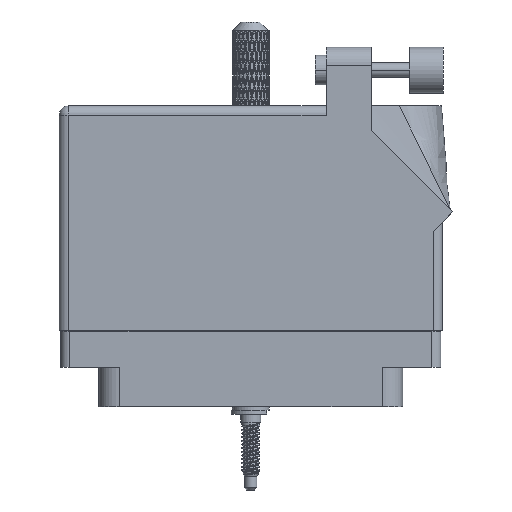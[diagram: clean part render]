
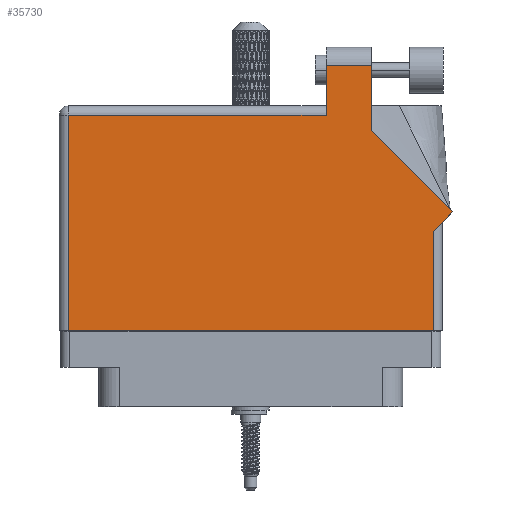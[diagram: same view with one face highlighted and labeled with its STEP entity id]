
A CAD part, front view. The second image highlights one B-rep face of the part: STEP entity #35730.
In plain terms, the highlighted face is planar.
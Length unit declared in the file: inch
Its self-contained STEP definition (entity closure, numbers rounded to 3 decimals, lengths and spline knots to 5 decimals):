
#461 = ORIENTED_EDGE ( 'NONE', *, *, #35735, .T. ) ;
#1427 = LINE ( 'NONE', #69661, #65424 ) ;
#1857 = CARTESIAN_POINT ( 'NONE',  ( -1.244, -0.1, 0.455 ) ) ;
#3035 = CARTESIAN_POINT ( 'NONE',  ( -1.306, 1.43, 0.455 ) ) ;
#3045 = VERTEX_POINT ( 'NONE', #46805 ) ;
#9714 = CARTESIAN_POINT ( 'NONE',  ( 0.513, 1.43, 0.455 ) ) ;
#10929 = VECTOR ( 'NONE', #101242, 39.37008 ) ;
#12456 = CARTESIAN_POINT ( 'NONE',  ( 1.244, 0.637, 0.455 ) ) ;
#15133 = VERTEX_POINT ( 'NONE', #17877 ) ;
#17607 = CARTESIAN_POINT ( 'NONE',  ( 1.37671, 0.70771, 0.455 ) ) ;
#17877 = CARTESIAN_POINT ( 'NONE',  ( 1.244, -0.1, 0.455 ) ) ;
#18217 = ORIENTED_EDGE ( 'NONE', *, *, #37475, .T. ) ;
#20458 = ORIENTED_EDGE ( 'NONE', *, *, #99227, .T. ) ;
#21428 = LINE ( 'NONE', #12456, #99549 ) ;
#21440 = DIRECTION ( 'NONE',  ( 0., 1., 0. ) ) ;
#21801 = LINE ( 'NONE', #76843, #89951 ) ;
#21829 = CARTESIAN_POINT ( 'NONE',  ( 0.82, 1.26442, 0.455 ) ) ;
#22367 = CARTESIAN_POINT ( 'NONE',  ( -1.244, 1.368, 0.455 ) ) ;
#26909 = LINE ( 'NONE', #9714, #49633 ) ;
#35700 = VECTOR ( 'NONE', #84790, 39.37008 ) ;
#35730 = ADVANCED_FACE ( 'NONE', ( #83918 ), #110206, .F. ) ;
#35735 = EDGE_CURVE ( 'NONE', #67840, #49804, #72578, .T. ) ;
#36188 = EDGE_CURVE ( 'NONE', #3045, #116343, #1427, .T. ) ;
#36467 = EDGE_CURVE ( 'NONE', #81797, #103691, #62552, .T. ) ;
#37475 = EDGE_CURVE ( 'NONE', #96140, #67840, #86640, .T. ) ;
#37841 = ORIENTED_EDGE ( 'NONE', *, *, #52600, .T. ) ;
#38624 = EDGE_CURVE ( 'NONE', #116343, #96140, #26909, .T. ) ;
#44451 = ORIENTED_EDGE ( 'NONE', *, *, #36467, .T. ) ;
#46805 = CARTESIAN_POINT ( 'NONE',  ( 0.82, 1.705, 0.455 ) ) ;
#49584 = EDGE_LOOP ( 'NONE', ( #85279, #93292, #104992, #18217, #461, #37841, #75989, #44451, #20458 ) ) ;
#49633 = VECTOR ( 'NONE', #86597, 39.37008 ) ;
#49804 = VERTEX_POINT ( 'NONE', #97692 ) ;
#51833 = LINE ( 'NONE', #21829, #105667 ) ;
#52600 = EDGE_CURVE ( 'NONE', #49804, #15133, #21801, .T. ) ;
#55684 = CARTESIAN_POINT ( 'NONE',  ( 1.37671, 0.70771, 0.455 ) ) ;
#57481 = DIRECTION ( 'NONE',  ( 0., 0., -1. ) ) ;
#59313 = DIRECTION ( 'NONE',  ( -1., 0., 0. ) ) ;
#61308 = DIRECTION ( 'NONE',  ( -1., 0., 0. ) ) ;
#61476 = CARTESIAN_POINT ( 'NONE',  ( 0.82, 1.26442, 0.455 ) ) ;
#62552 = LINE ( 'NONE', #65474, #83809 ) ;
#65055 = DIRECTION ( 'NONE',  ( 0.707, 0.707, 0. ) ) ;
#65424 = VECTOR ( 'NONE', #61308, 39.37008 ) ;
#65474 = CARTESIAN_POINT ( 'NONE',  ( 1.306, 0.637, 0.455 ) ) ;
#65504 = CARTESIAN_POINT ( 'NONE',  ( 0.513, 1.368, 0.455 ) ) ;
#67840 = VERTEX_POINT ( 'NONE', #22367 ) ;
#69661 = CARTESIAN_POINT ( 'NONE',  ( 0.513, 1.705, 0.455 ) ) ;
#72578 = LINE ( 'NONE', #1857, #35700 ) ;
#75989 = ORIENTED_EDGE ( 'NONE', *, *, #111049, .T. ) ;
#76843 = CARTESIAN_POINT ( 'NONE',  ( -1.306, -0.1, 0.455 ) ) ;
#81797 = VERTEX_POINT ( 'NONE', #107745 ) ;
#83809 = VECTOR ( 'NONE', #65055, 39.37008 ) ;
#83918 = FACE_OUTER_BOUND ( 'NONE', #49584, .T. ) ;
#84409 = DIRECTION ( 'NONE',  ( -1., 0., 0. ) ) ;
#84790 = DIRECTION ( 'NONE',  ( 0., -1., 0. ) ) ;
#85279 = ORIENTED_EDGE ( 'NONE', *, *, #101609, .T. ) ;
#86233 = CARTESIAN_POINT ( 'NONE',  ( -1.306, 1.368, 0.455 ) ) ;
#86597 = DIRECTION ( 'NONE',  ( 0., -1., 0. ) ) ;
#86640 = LINE ( 'NONE', #86233, #100892 ) ;
#89951 = VECTOR ( 'NONE', #95101, 39.37008 ) ;
#93292 = ORIENTED_EDGE ( 'NONE', *, *, #36188, .T. ) ;
#95101 = DIRECTION ( 'NONE',  ( 1., 0., 0. ) ) ;
#95185 = VERTEX_POINT ( 'NONE', #61476 ) ;
#96140 = VERTEX_POINT ( 'NONE', #65504 ) ;
#97692 = CARTESIAN_POINT ( 'NONE',  ( -1.244, -0.1, 0.455 ) ) ;
#99227 = EDGE_CURVE ( 'NONE', #103691, #95185, #106114, .T. ) ;
#99549 = VECTOR ( 'NONE', #112079, 39.37008 ) ;
#100892 = VECTOR ( 'NONE', #59313, 39.37008 ) ;
#101242 = DIRECTION ( 'NONE',  ( -0.707, 0.707, 0. ) ) ;
#101609 = EDGE_CURVE ( 'NONE', #95185, #3045, #51833, .T. ) ;
#103691 = VERTEX_POINT ( 'NONE', #17607 ) ;
#104992 = ORIENTED_EDGE ( 'NONE', *, *, #38624, .T. ) ;
#105166 = AXIS2_PLACEMENT_3D ( 'NONE', #3035, #57481, #84409 ) ;
#105667 = VECTOR ( 'NONE', #21440, 39.37008 ) ;
#106114 = LINE ( 'NONE', #55684, #10929 ) ;
#107745 = CARTESIAN_POINT ( 'NONE',  ( 1.244, 0.575, 0.455 ) ) ;
#110206 = PLANE ( 'NONE',  #105166 ) ;
#110842 = CARTESIAN_POINT ( 'NONE',  ( 0.513, 1.705, 0.455 ) ) ;
#111049 = EDGE_CURVE ( 'NONE', #15133, #81797, #21428, .T. ) ;
#112079 = DIRECTION ( 'NONE',  ( 0., 1., 0. ) ) ;
#116343 = VERTEX_POINT ( 'NONE', #110842 ) ;
